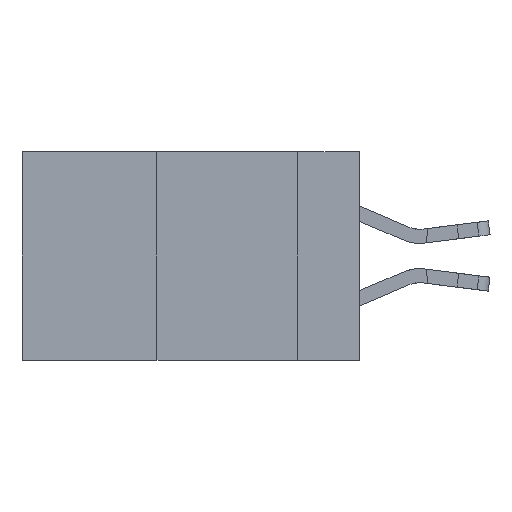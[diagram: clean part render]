
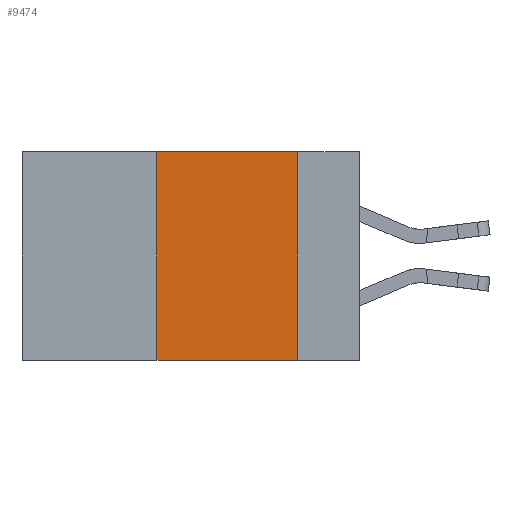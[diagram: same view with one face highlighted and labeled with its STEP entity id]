
A CAD part, left-side view. The second image highlights one B-rep face of the part: STEP entity #9474.
In plain terms, the highlighted planar face has unit normal (-1, 0, 0).
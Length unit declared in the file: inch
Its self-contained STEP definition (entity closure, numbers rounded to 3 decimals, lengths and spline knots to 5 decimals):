
#207 = LINE ( 'NONE', #1986, #18307 ) ;
#422 = ORIENTED_EDGE ( 'NONE', *, *, #18297, .F. ) ;
#657 = VERTEX_POINT ( 'NONE', #17059 ) ;
#1986 = CARTESIAN_POINT ( 'NONE',  ( 0., 0.6, -0.37 ) ) ;
#2147 = LINE ( 'NONE', #5075, #5083 ) ;
#2601 = VERTEX_POINT ( 'NONE', #7463 ) ;
#3702 = CARTESIAN_POINT ( 'NONE',  ( 0., 0.6, 0. ) ) ;
#4995 = VERTEX_POINT ( 'NONE', #9440 ) ;
#5075 = CARTESIAN_POINT ( 'NONE',  ( 0., 0.11, 0. ) ) ;
#5083 = VECTOR ( 'NONE', #17307, 39.37008 ) ;
#7463 = CARTESIAN_POINT ( 'NONE',  ( 0., 0.36, -0.37 ) ) ;
#8409 = LINE ( 'NONE', #10111, #18506 ) ;
#8456 = VECTOR ( 'NONE', #15380, 39.37008 ) ;
#8697 = EDGE_CURVE ( 'NONE', #15852, #657, #2147, .T. ) ;
#8940 = DIRECTION ( 'NONE',  ( 0., -1., 0. ) ) ;
#9440 = CARTESIAN_POINT ( 'NONE',  ( 0., 0.36, 0. ) ) ;
#9474 = ADVANCED_FACE ( 'NONE', ( #9743 ), #16685, .F. ) ;
#9743 = FACE_OUTER_BOUND ( 'NONE', #17349, .T. ) ;
#10111 = CARTESIAN_POINT ( 'NONE',  ( 0., 0.36, 0. ) ) ;
#13087 = ORIENTED_EDGE ( 'NONE', *, *, #20759, .F. ) ;
#15380 = DIRECTION ( 'NONE',  ( 0., -1., 0. ) ) ;
#15499 = LINE ( 'NONE', #3702, #8456 ) ;
#15710 = EDGE_CURVE ( 'NONE', #2601, #657, #207, .T. ) ;
#15852 = VERTEX_POINT ( 'NONE', #16442 ) ;
#16442 = CARTESIAN_POINT ( 'NONE',  ( 0., 0.11, 0. ) ) ;
#16685 = PLANE ( 'NONE',  #17277 ) ;
#17059 = CARTESIAN_POINT ( 'NONE',  ( 0., 0.11, -0.37 ) ) ;
#17277 = AXIS2_PLACEMENT_3D ( 'NONE', #18049, #21857, #20174 ) ;
#17307 = DIRECTION ( 'NONE',  ( 0., 0., -1. ) ) ;
#17349 = EDGE_LOOP ( 'NONE', ( #20401, #422, #13087, #18350 ) ) ;
#18049 = CARTESIAN_POINT ( 'NONE',  ( 0., 0.6, 0. ) ) ;
#18297 = EDGE_CURVE ( 'NONE', #4995, #15852, #15499, .T. ) ;
#18307 = VECTOR ( 'NONE', #8940, 39.37008 ) ;
#18350 = ORIENTED_EDGE ( 'NONE', *, *, #15710, .T. ) ;
#18506 = VECTOR ( 'NONE', #21887, 39.37008 ) ;
#20174 = DIRECTION ( 'NONE',  ( 0., 0., -1. ) ) ;
#20401 = ORIENTED_EDGE ( 'NONE', *, *, #8697, .F. ) ;
#20759 = EDGE_CURVE ( 'NONE', #2601, #4995, #8409, .T. ) ;
#21857 = DIRECTION ( 'NONE',  ( 1., 0., 0. ) ) ;
#21887 = DIRECTION ( 'NONE',  ( 0., 0., 1. ) ) ;
